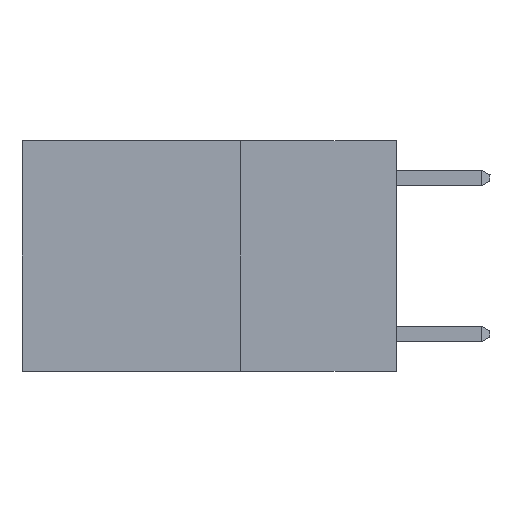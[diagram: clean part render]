
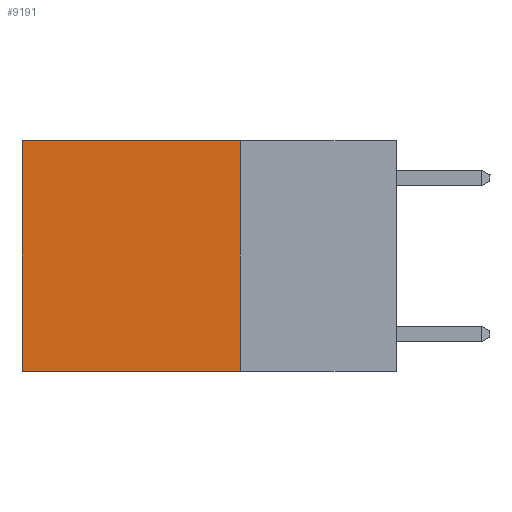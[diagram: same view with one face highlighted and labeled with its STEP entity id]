
A CAD part, left-side view. The second image highlights one B-rep face of the part: STEP entity #9191.
In plain terms, the highlighted planar face has unit normal (-1, 0, 0).
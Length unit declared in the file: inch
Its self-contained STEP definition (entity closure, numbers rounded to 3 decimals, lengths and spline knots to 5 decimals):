
#162 = DIRECTION ( 'NONE',  ( 0., 1., 0. ) ) ;
#213 = FACE_OUTER_BOUND ( 'NONE', #7793, .T. ) ;
#1036 = CARTESIAN_POINT ( 'NONE',  ( 0.2625, 0.25, 0. ) ) ;
#1328 = LINE ( 'NONE', #3827, #9517 ) ;
#1782 = VECTOR ( 'NONE', #162, 39.37008 ) ;
#1954 = VERTEX_POINT ( 'NONE', #4855 ) ;
#2171 = CARTESIAN_POINT ( 'NONE',  ( 0.2625, 0.25, -0.37 ) ) ;
#2612 = DIRECTION ( 'NONE',  ( 0., 1., 0. ) ) ;
#2645 = VECTOR ( 'NONE', #2612, 39.37008 ) ;
#3515 = LINE ( 'NONE', #4900, #1782 ) ;
#3827 = CARTESIAN_POINT ( 'NONE',  ( 0.2625, 0.6, 0. ) ) ;
#4112 = CARTESIAN_POINT ( 'NONE',  ( 0.2625, 0.25, -0.37 ) ) ;
#4203 = ORIENTED_EDGE ( 'NONE', *, *, #4877, .T. ) ;
#4261 = CARTESIAN_POINT ( 'NONE',  ( 0.2625, 0.25, 0. ) ) ;
#4349 = PLANE ( 'NONE',  #4632 ) ;
#4416 = EDGE_CURVE ( 'NONE', #9046, #6216, #9015, .T. ) ;
#4632 = AXIS2_PLACEMENT_3D ( 'NONE', #6741, #5785, #9809 ) ;
#4647 = DIRECTION ( 'NONE',  ( 0., 0., -1. ) ) ;
#4855 = CARTESIAN_POINT ( 'NONE',  ( 0.2625, 0.6, 0. ) ) ;
#4877 = EDGE_CURVE ( 'NONE', #1954, #6740, #1328, .T. ) ;
#4900 = CARTESIAN_POINT ( 'NONE',  ( 0.2625, 0.25, 0. ) ) ;
#5726 = EDGE_CURVE ( 'NONE', #9046, #1954, #3515, .T. ) ;
#5752 = DIRECTION ( 'NONE',  ( 0., 0., -1. ) ) ;
#5785 = DIRECTION ( 'NONE',  ( 1., 0., 0. ) ) ;
#6216 = VERTEX_POINT ( 'NONE', #2171 ) ;
#6368 = ORIENTED_EDGE ( 'NONE', *, *, #4416, .F. ) ;
#6740 = VERTEX_POINT ( 'NONE', #7494 ) ;
#6741 = CARTESIAN_POINT ( 'NONE',  ( 0.2625, 0.25, 0. ) ) ;
#7117 = EDGE_CURVE ( 'NONE', #6216, #6740, #8014, .T. ) ;
#7494 = CARTESIAN_POINT ( 'NONE',  ( 0.2625, 0.6, -0.37 ) ) ;
#7793 = EDGE_LOOP ( 'NONE', ( #4203, #10048, #6368, #10165 ) ) ;
#8014 = LINE ( 'NONE', #4112, #2645 ) ;
#9015 = LINE ( 'NONE', #1036, #10182 ) ;
#9046 = VERTEX_POINT ( 'NONE', #4261 ) ;
#9191 = ADVANCED_FACE ( 'NONE', ( #213 ), #4349, .F. ) ;
#9517 = VECTOR ( 'NONE', #4647, 39.37008 ) ;
#9809 = DIRECTION ( 'NONE',  ( 0., 0., -1. ) ) ;
#10048 = ORIENTED_EDGE ( 'NONE', *, *, #7117, .F. ) ;
#10165 = ORIENTED_EDGE ( 'NONE', *, *, #5726, .T. ) ;
#10182 = VECTOR ( 'NONE', #5752, 39.37008 ) ;
